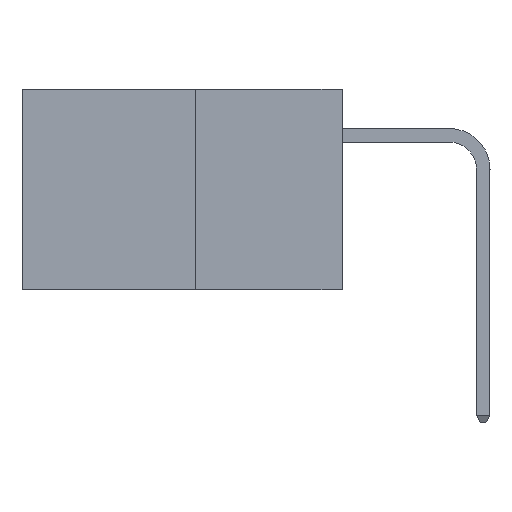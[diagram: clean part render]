
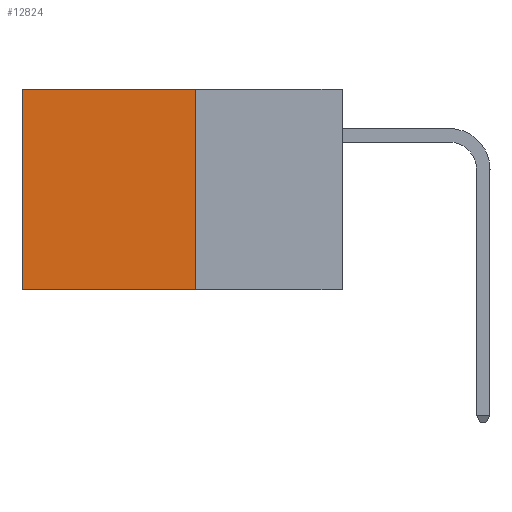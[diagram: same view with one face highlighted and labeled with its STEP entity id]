
A CAD part, left-side view. The second image highlights one B-rep face of the part: STEP entity #12824.
In plain terms, the highlighted planar face has unit normal (-1, 0, 0).
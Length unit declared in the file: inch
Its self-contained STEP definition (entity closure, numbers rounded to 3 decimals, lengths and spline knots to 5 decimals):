
#185 = CARTESIAN_POINT ( 'NONE',  ( 0.277, 0.27, -0.37 ) ) ;
#232 = ORIENTED_EDGE ( 'NONE', *, *, #2849, .F. ) ;
#435 = VERTEX_POINT ( 'NONE', #185 ) ;
#528 = CARTESIAN_POINT ( 'NONE',  ( 0.277, 0.27, 0. ) ) ;
#556 = CARTESIAN_POINT ( 'NONE',  ( 0.277, 0.59, -0.37 ) ) ;
#928 = DIRECTION ( 'NONE',  ( 1., 0., 0. ) ) ;
#1812 = DIRECTION ( 'NONE',  ( 0., 1., 0. ) ) ;
#2286 = EDGE_CURVE ( 'NONE', #3708, #13703, #6065, .T. ) ;
#2575 = DIRECTION ( 'NONE',  ( 0., 0., -1. ) ) ;
#2726 = AXIS2_PLACEMENT_3D ( 'NONE', #15477, #928, #9599 ) ;
#2849 = EDGE_CURVE ( 'NONE', #14753, #435, #7029, .T. ) ;
#3364 = DIRECTION ( 'NONE',  ( 0., 0., -1. ) ) ;
#3627 = ORIENTED_EDGE ( 'NONE', *, *, #4204, .T. ) ;
#3708 = VERTEX_POINT ( 'NONE', #4536 ) ;
#3746 = DIRECTION ( 'NONE',  ( 0., 1., 0. ) ) ;
#4204 = EDGE_CURVE ( 'NONE', #14753, #3708, #10654, .T. ) ;
#4536 = CARTESIAN_POINT ( 'NONE',  ( 0.277, 0.59, 0. ) ) ;
#5671 = VECTOR ( 'NONE', #3364, 39.37008 ) ;
#5883 = EDGE_LOOP ( 'NONE', ( #11521, #12935, #232, #3627 ) ) ;
#6065 = LINE ( 'NONE', #8862, #5671 ) ;
#7029 = LINE ( 'NONE', #7983, #13417 ) ;
#7588 = FACE_OUTER_BOUND ( 'NONE', #5883, .T. ) ;
#7983 = CARTESIAN_POINT ( 'NONE',  ( 0.277, 0.27, -0.37 ) ) ;
#8074 = LINE ( 'NONE', #11055, #14064 ) ;
#8755 = EDGE_CURVE ( 'NONE', #435, #13703, #8074, .T. ) ;
#8862 = CARTESIAN_POINT ( 'NONE',  ( 0.277, 0.59, -0.37 ) ) ;
#9599 = DIRECTION ( 'NONE',  ( 0., 0., -1. ) ) ;
#10278 = VECTOR ( 'NONE', #1812, 39.37008 ) ;
#10654 = LINE ( 'NONE', #528, #10278 ) ;
#11055 = CARTESIAN_POINT ( 'NONE',  ( 0.277, 0.27, -0.37 ) ) ;
#11148 = CARTESIAN_POINT ( 'NONE',  ( 0.277, 0.27, 0. ) ) ;
#11521 = ORIENTED_EDGE ( 'NONE', *, *, #2286, .T. ) ;
#12824 = ADVANCED_FACE ( 'NONE', ( #7588 ), #14314, .F. ) ;
#12935 = ORIENTED_EDGE ( 'NONE', *, *, #8755, .F. ) ;
#13417 = VECTOR ( 'NONE', #2575, 39.37008 ) ;
#13703 = VERTEX_POINT ( 'NONE', #556 ) ;
#14064 = VECTOR ( 'NONE', #3746, 39.37008 ) ;
#14314 = PLANE ( 'NONE',  #2726 ) ;
#14753 = VERTEX_POINT ( 'NONE', #11148 ) ;
#15477 = CARTESIAN_POINT ( 'NONE',  ( 0.277, 0.27, -0.37 ) ) ;
